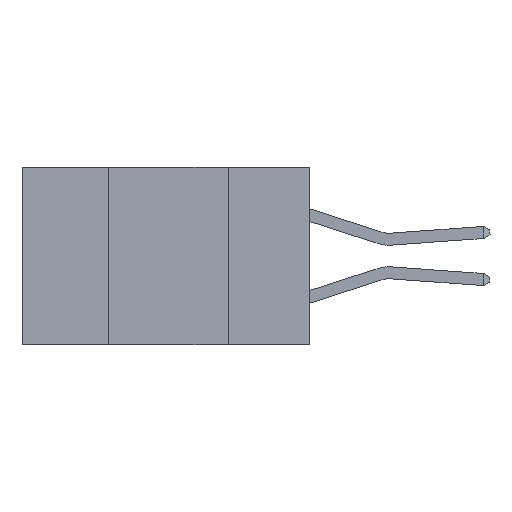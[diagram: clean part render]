
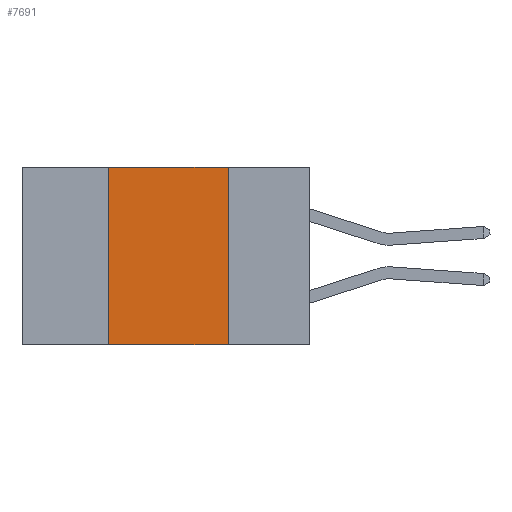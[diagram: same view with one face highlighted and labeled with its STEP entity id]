
A CAD part, left-side view. The second image highlights one B-rep face of the part: STEP entity #7691.
In plain terms, the highlighted planar face has unit normal (-1, 0, 0).
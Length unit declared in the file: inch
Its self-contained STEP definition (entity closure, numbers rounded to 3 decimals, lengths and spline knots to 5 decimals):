
#230 = ORIENTED_EDGE ( 'NONE', *, *, #1417, .F. ) ;
#715 = AXIS2_PLACEMENT_3D ( 'NONE', #6889, #7824, #1703 ) ;
#943 = ORIENTED_EDGE ( 'NONE', *, *, #2791, .F. ) ;
#1016 = CARTESIAN_POINT ( 'NONE',  ( 0., 0.42, -0.37 ) ) ;
#1417 = EDGE_CURVE ( 'NONE', #6795, #3536, #7433, .T. ) ;
#1694 = LINE ( 'NONE', #7457, #11771 ) ;
#1703 = DIRECTION ( 'NONE',  ( 0., 0., -1. ) ) ;
#2005 = VECTOR ( 'NONE', #9254, 39.37008 ) ;
#2303 = EDGE_CURVE ( 'NONE', #6145, #12630, #4977, .T. ) ;
#2313 = VECTOR ( 'NONE', #2448, 39.37008 ) ;
#2448 = DIRECTION ( 'NONE',  ( 0., 0., -1. ) ) ;
#2545 = CARTESIAN_POINT ( 'NONE',  ( 0., 0.17, -0.37 ) ) ;
#2791 = EDGE_CURVE ( 'NONE', #3536, #12630, #12520, .T. ) ;
#3246 = EDGE_CURVE ( 'NONE', #6145, #6795, #1694, .T. ) ;
#3536 = VERTEX_POINT ( 'NONE', #7921 ) ;
#4395 = ORIENTED_EDGE ( 'NONE', *, *, #2303, .T. ) ;
#4977 = LINE ( 'NONE', #9878, #12132 ) ;
#6145 = VERTEX_POINT ( 'NONE', #1016 ) ;
#6447 = ORIENTED_EDGE ( 'NONE', *, *, #3246, .F. ) ;
#6550 = CARTESIAN_POINT ( 'NONE',  ( 0., 0.17, 0. ) ) ;
#6795 = VERTEX_POINT ( 'NONE', #6908 ) ;
#6889 = CARTESIAN_POINT ( 'NONE',  ( 0., 0.6, 0. ) ) ;
#6908 = CARTESIAN_POINT ( 'NONE',  ( 0., 0.42, 0. ) ) ;
#6971 = FACE_OUTER_BOUND ( 'NONE', #10967, .T. ) ;
#7433 = LINE ( 'NONE', #8526, #2005 ) ;
#7457 = CARTESIAN_POINT ( 'NONE',  ( 0., 0.42, 0. ) ) ;
#7691 = ADVANCED_FACE ( 'NONE', ( #6971 ), #12352, .F. ) ;
#7824 = DIRECTION ( 'NONE',  ( 1., 0., 0. ) ) ;
#7921 = CARTESIAN_POINT ( 'NONE',  ( 0., 0.17, 0. ) ) ;
#8526 = CARTESIAN_POINT ( 'NONE',  ( 0., 0.6, 0. ) ) ;
#9254 = DIRECTION ( 'NONE',  ( 0., -1., 0. ) ) ;
#9878 = CARTESIAN_POINT ( 'NONE',  ( 0., 0.6, -0.37 ) ) ;
#10967 = EDGE_LOOP ( 'NONE', ( #943, #230, #6447, #4395 ) ) ;
#11771 = VECTOR ( 'NONE', #12413, 39.37008 ) ;
#12132 = VECTOR ( 'NONE', #12755, 39.37008 ) ;
#12352 = PLANE ( 'NONE',  #715 ) ;
#12413 = DIRECTION ( 'NONE',  ( 0., 0., 1. ) ) ;
#12520 = LINE ( 'NONE', #6550, #2313 ) ;
#12630 = VERTEX_POINT ( 'NONE', #2545 ) ;
#12755 = DIRECTION ( 'NONE',  ( 0., -1., 0. ) ) ;
